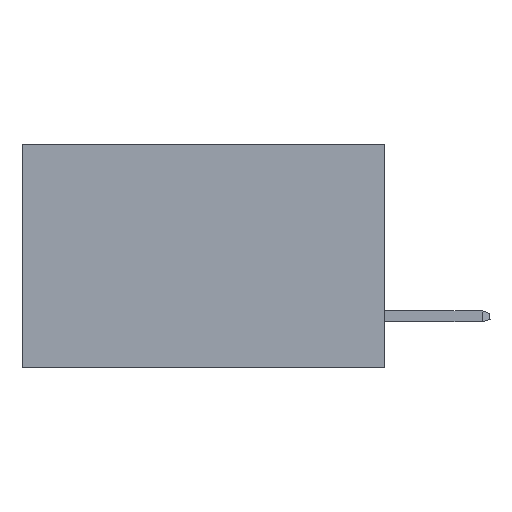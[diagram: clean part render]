
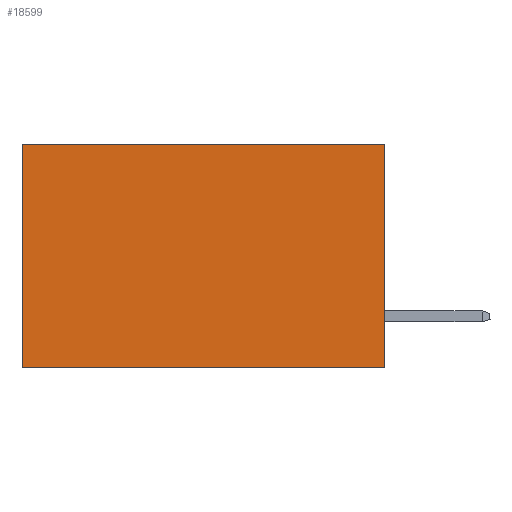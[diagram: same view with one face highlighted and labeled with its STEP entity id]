
A CAD part, left-side view. The second image highlights one B-rep face of the part: STEP entity #18599.
In plain terms, the highlighted planar face has unit normal (-1, 0, 0).
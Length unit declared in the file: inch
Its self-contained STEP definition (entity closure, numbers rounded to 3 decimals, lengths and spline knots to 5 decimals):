
#1251 = DIRECTION ( 'NONE',  ( 0., 0., -1. ) ) ;
#1696 = LINE ( 'NONE', #19279, #9701 ) ;
#1802 = EDGE_LOOP ( 'NONE', ( #4963, #7335, #14449, #21340 ) ) ;
#3217 = FACE_OUTER_BOUND ( 'NONE', #1802, .T. ) ;
#3763 = DIRECTION ( 'NONE',  ( 0., 0., -1. ) ) ;
#4963 = ORIENTED_EDGE ( 'NONE', *, *, #4989, .T. ) ;
#4989 = EDGE_CURVE ( 'NONE', #14277, #7175, #13356, .T. ) ;
#5729 = DIRECTION ( 'NONE',  ( 1., 0., 0. ) ) ;
#5735 = VECTOR ( 'NONE', #1251, 39.37008 ) ;
#7175 = VERTEX_POINT ( 'NONE', #23354 ) ;
#7335 = ORIENTED_EDGE ( 'NONE', *, *, #18898, .F. ) ;
#7349 = DIRECTION ( 'NONE',  ( 0., 1., 0. ) ) ;
#9364 = EDGE_CURVE ( 'NONE', #19414, #14277, #1696, .T. ) ;
#9701 = VECTOR ( 'NONE', #7349, 39.37008 ) ;
#9799 = CARTESIAN_POINT ( 'NONE',  ( 0.298, 0., -0.37 ) ) ;
#9982 = VECTOR ( 'NONE', #14365, 39.37008 ) ;
#10042 = AXIS2_PLACEMENT_3D ( 'NONE', #11707, #5729, #3763 ) ;
#11384 = CARTESIAN_POINT ( 'NONE',  ( 0.298, 0., 0. ) ) ;
#11594 = VERTEX_POINT ( 'NONE', #9799 ) ;
#11707 = CARTESIAN_POINT ( 'NONE',  ( 0.298, 0., 0. ) ) ;
#12308 = CARTESIAN_POINT ( 'NONE',  ( 0.298, 0., -0.37 ) ) ;
#13087 = CARTESIAN_POINT ( 'NONE',  ( 0.298, 0.6, 0. ) ) ;
#13356 = LINE ( 'NONE', #19796, #23208 ) ;
#14135 = EDGE_CURVE ( 'NONE', #19414, #11594, #23642, .T. ) ;
#14277 = VERTEX_POINT ( 'NONE', #13087 ) ;
#14365 = DIRECTION ( 'NONE',  ( 0., 1., 0. ) ) ;
#14449 = ORIENTED_EDGE ( 'NONE', *, *, #14135, .F. ) ;
#15761 = PLANE ( 'NONE',  #10042 ) ;
#18599 = ADVANCED_FACE ( 'NONE', ( #3217 ), #15761, .F. ) ;
#18898 = EDGE_CURVE ( 'NONE', #11594, #7175, #24481, .T. ) ;
#19279 = CARTESIAN_POINT ( 'NONE',  ( 0.298, 0., 0. ) ) ;
#19414 = VERTEX_POINT ( 'NONE', #11384 ) ;
#19796 = CARTESIAN_POINT ( 'NONE',  ( 0.298, 0.6, 0. ) ) ;
#21340 = ORIENTED_EDGE ( 'NONE', *, *, #9364, .T. ) ;
#23208 = VECTOR ( 'NONE', #23390, 39.37008 ) ;
#23354 = CARTESIAN_POINT ( 'NONE',  ( 0.298, 0.6, -0.37 ) ) ;
#23390 = DIRECTION ( 'NONE',  ( 0., 0., -1. ) ) ;
#23642 = LINE ( 'NONE', #24667, #5735 ) ;
#24481 = LINE ( 'NONE', #12308, #9982 ) ;
#24667 = CARTESIAN_POINT ( 'NONE',  ( 0.298, 0., 0. ) ) ;
